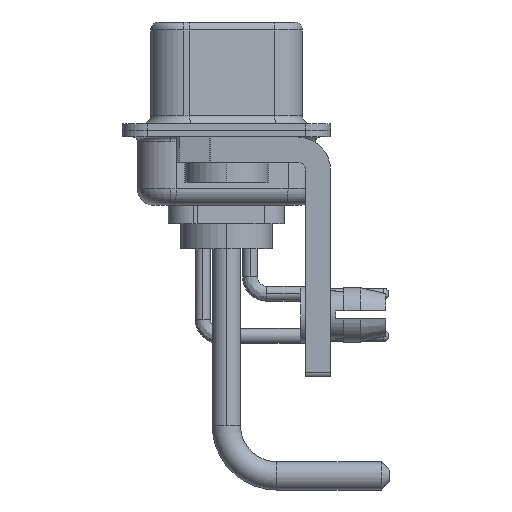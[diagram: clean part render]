
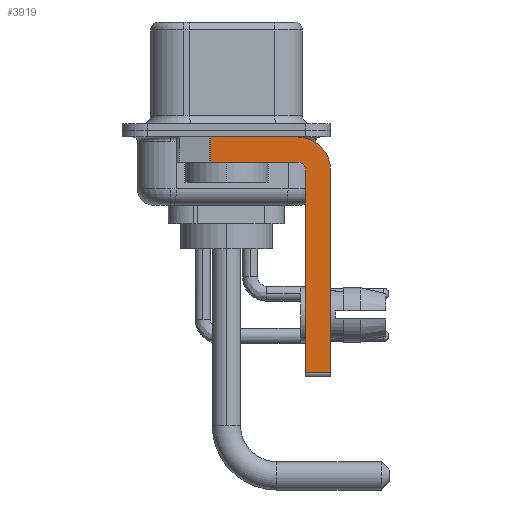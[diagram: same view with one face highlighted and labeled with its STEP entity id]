
A CAD part, left-side view. The second image highlights one B-rep face of the part: STEP entity #3919.
In plain terms, the highlighted planar face has unit normal (-1, 0, 0).
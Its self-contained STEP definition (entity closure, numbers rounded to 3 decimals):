
#612 = VECTOR ( 'NONE', #696, 1000. ) ;
#696 = DIRECTION ( 'NONE',  ( 0., 1., 0. ) ) ;
#743 = DIRECTION ( 'NONE',  ( 1., 0., 0. ) ) ;
#894 = CARTESIAN_POINT ( 'NONE',  ( -2.9, -6.25, -2.4 ) ) ;
#1436 = LINE ( 'NONE', #7525, #15773 ) ;
#1621 = CARTESIAN_POINT ( 'NONE',  ( -2.9, 0.978, -1.9 ) ) ;
#2244 = DIRECTION ( 'NONE',  ( 0., -1., 0. ) ) ;
#2282 = EDGE_CURVE ( 'NONE', #22773, #13162, #26184, .T. ) ;
#2353 = EDGE_CURVE ( 'NONE', #6632, #8579, #3064, .T. ) ;
#3008 = EDGE_CURVE ( 'NONE', #14971, #6632, #6400, .T. ) ;
#3064 = CIRCLE ( 'NONE', #18112, 2. ) ;
#3893 = ORIENTED_EDGE ( 'NONE', *, *, #6122, .F. ) ;
#3919 = ADVANCED_FACE ( 'NONE', ( #4901 ), #5311, .F. ) ;
#4036 = EDGE_CURVE ( 'NONE', #8579, #13162, #1436, .T. ) ;
#4158 = VERTEX_POINT ( 'NONE', #21309 ) ;
#4317 = CARTESIAN_POINT ( 'NONE',  ( -2.9, 3., -0.4 ) ) ;
#4901 = FACE_OUTER_BOUND ( 'NONE', #25250, .T. ) ;
#4934 = CARTESIAN_POINT ( 'NONE',  ( -2.9, -4.25, -2.4 ) ) ;
#5311 = PLANE ( 'NONE',  #14891 ) ;
#5718 = VECTOR ( 'NONE', #9494, 1000. ) ;
#6122 = EDGE_CURVE ( 'NONE', #22773, #23286, #24912, .T. ) ;
#6400 = LINE ( 'NONE', #4317, #6541 ) ;
#6541 = VECTOR ( 'NONE', #2244, 1000. ) ;
#6609 = ORIENTED_EDGE ( 'NONE', *, *, #4036, .F. ) ;
#6632 = VERTEX_POINT ( 'NONE', #23313 ) ;
#7028 = CARTESIAN_POINT ( 'NONE',  ( -2.9, -4.75, -2.4 ) ) ;
#7320 = EDGE_CURVE ( 'NONE', #23286, #4158, #24216, .T. ) ;
#7525 = CARTESIAN_POINT ( 'NONE',  ( -2.9, -6.25, -2.4 ) ) ;
#7702 = ORIENTED_EDGE ( 'NONE', *, *, #2353, .F. ) ;
#8159 = EDGE_CURVE ( 'NONE', #14971, #8681, #9546, .T. ) ;
#8579 = VERTEX_POINT ( 'NONE', #894 ) ;
#8681 = VERTEX_POINT ( 'NONE', #26586 ) ;
#8909 = DIRECTION ( 'NONE',  ( 0., 0., -1. ) ) ;
#9012 = LINE ( 'NONE', #11103, #612 ) ;
#9264 = VECTOR ( 'NONE', #10069, 1000. ) ;
#9494 = DIRECTION ( 'NONE',  ( 0., -1., 0. ) ) ;
#9546 = LINE ( 'NONE', #1621, #9264 ) ;
#10069 = DIRECTION ( 'NONE',  ( 0., 0., -1. ) ) ;
#11103 = CARTESIAN_POINT ( 'NONE',  ( -2.9, -4.25, -1.9 ) ) ;
#11840 = DIRECTION ( 'NONE',  ( 0., 0., 1. ) ) ;
#12336 = AXIS2_PLACEMENT_3D ( 'NONE', #17915, #18324, #11840 ) ;
#12370 = DIRECTION ( 'NONE',  ( 0., 0., 1. ) ) ;
#13162 = VERTEX_POINT ( 'NONE', #25259 ) ;
#13373 = DIRECTION ( 'NONE',  ( 0., 0., -1. ) ) ;
#14443 = CARTESIAN_POINT ( 'NONE',  ( -2.9, -4.75, -14.8 ) ) ;
#14703 = ORIENTED_EDGE ( 'NONE', *, *, #8159, .T. ) ;
#14891 = AXIS2_PLACEMENT_3D ( 'NONE', #23960, #743, #8909 ) ;
#14971 = VERTEX_POINT ( 'NONE', #21890 ) ;
#15225 = EDGE_CURVE ( 'NONE', #4158, #8681, #9012, .T. ) ;
#15362 = VECTOR ( 'NONE', #12370, 1000. ) ;
#15773 = VECTOR ( 'NONE', #26561, 1000. ) ;
#17259 = ORIENTED_EDGE ( 'NONE', *, *, #2282, .T. ) ;
#17461 = ORIENTED_EDGE ( 'NONE', *, *, #15225, .F. ) ;
#17915 = CARTESIAN_POINT ( 'NONE',  ( -2.9, -4.25, -2.4 ) ) ;
#18112 = AXIS2_PLACEMENT_3D ( 'NONE', #4934, #21505, #13373 ) ;
#18324 = DIRECTION ( 'NONE',  ( -1., 0., 0. ) ) ;
#20005 = CARTESIAN_POINT ( 'NONE',  ( -2.9, -4.25, -14.55 ) ) ;
#21309 = CARTESIAN_POINT ( 'NONE',  ( -2.9, -4.25, -1.9 ) ) ;
#21505 = DIRECTION ( 'NONE',  ( 1., 0., 0. ) ) ;
#21890 = CARTESIAN_POINT ( 'NONE',  ( -2.9, 0.978, -0.4 ) ) ;
#22773 = VERTEX_POINT ( 'NONE', #26095 ) ;
#23286 = VERTEX_POINT ( 'NONE', #7028 ) ;
#23313 = CARTESIAN_POINT ( 'NONE',  ( -2.9, -4.25, -0.4 ) ) ;
#23960 = CARTESIAN_POINT ( 'NONE',  ( -2.9, -4.25, -2.4 ) ) ;
#24216 = CIRCLE ( 'NONE', #12336, 0.5 ) ;
#24263 = ORIENTED_EDGE ( 'NONE', *, *, #7320, .F. ) ;
#24912 = LINE ( 'NONE', #14443, #15362 ) ;
#25250 = EDGE_LOOP ( 'NONE', ( #26766, #14703, #17461, #24263, #3893, #17259, #6609, #7702 ) ) ;
#25259 = CARTESIAN_POINT ( 'NONE',  ( -2.9, -6.25, -14.55 ) ) ;
#26095 = CARTESIAN_POINT ( 'NONE',  ( -2.9, -4.75, -14.55 ) ) ;
#26184 = LINE ( 'NONE', #20005, #5718 ) ;
#26561 = DIRECTION ( 'NONE',  ( 0., 0., -1. ) ) ;
#26586 = CARTESIAN_POINT ( 'NONE',  ( -2.9, 0.978, -1.9 ) ) ;
#26766 = ORIENTED_EDGE ( 'NONE', *, *, #3008, .F. ) ;
